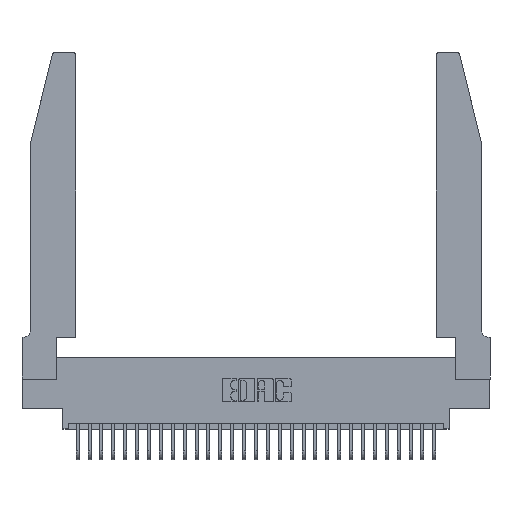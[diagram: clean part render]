
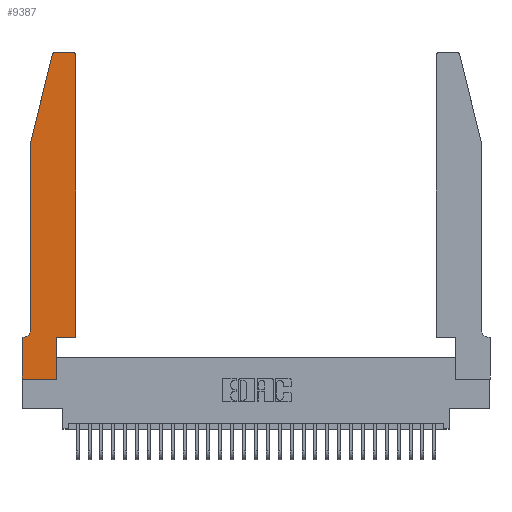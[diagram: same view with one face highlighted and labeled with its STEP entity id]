
A CAD part, top view. The second image highlights one B-rep face of the part: STEP entity #9387.
In plain terms, the highlighted planar face has unit normal (0, 0, 1).
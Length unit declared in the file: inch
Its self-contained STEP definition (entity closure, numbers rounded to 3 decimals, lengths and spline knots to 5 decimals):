
#382 = DIRECTION ( 'NONE',  ( 1., 0., 0. ) ) ;
#825 = CARTESIAN_POINT ( 'NONE',  ( 0.2605, 2.75, 0.37 ) ) ;
#938 = ORIENTED_EDGE ( 'NONE', *, *, #24118, .T. ) ;
#1009 = LINE ( 'NONE', #17457, #20301 ) ;
#1211 = VERTEX_POINT ( 'NONE', #24984 ) ;
#1546 = VERTEX_POINT ( 'NONE', #30286 ) ;
#1888 = ORIENTED_EDGE ( 'NONE', *, *, #3503, .T. ) ;
#2112 = DIRECTION ( 'NONE',  ( 0., 0., -1. ) ) ;
#2207 = CARTESIAN_POINT ( 'NONE',  ( 0.0755, 2., 0.37 ) ) ;
#2732 = VERTEX_POINT ( 'NONE', #14739 ) ;
#3503 = EDGE_CURVE ( 'NONE', #20145, #19215, #1009, .T. ) ;
#3600 = ORIENTED_EDGE ( 'NONE', *, *, #26522, .T. ) ;
#4084 = DIRECTION ( 'NONE',  ( -0.239, -0.971, 0. ) ) ;
#4304 = LINE ( 'NONE', #28898, #10932 ) ;
#5076 = VERTEX_POINT ( 'NONE', #25615 ) ;
#5944 = DIRECTION ( 'NONE',  ( -1., 0., 0. ) ) ;
#6118 = DIRECTION ( 'NONE',  ( 1., 0., 0. ) ) ;
#7181 = ORIENTED_EDGE ( 'NONE', *, *, #22778, .T. ) ;
#7302 = CARTESIAN_POINT ( 'NONE',  ( 0.2865, 0.35, 0.37 ) ) ;
#7409 = LINE ( 'NONE', #26250, #19209 ) ;
#7454 = CARTESIAN_POINT ( 'NONE',  ( 0.284, 2.72, 0.37 ) ) ;
#7634 = EDGE_LOOP ( 'NONE', ( #18173, #3600, #7181, #1888, #30532, #29376, #14653, #9561, #26507, #25388, #938, #20153 ) ) ;
#9213 = AXIS2_PLACEMENT_3D ( 'NONE', #17176, #2112, #19725 ) ;
#9292 = LINE ( 'NONE', #7302, #22596 ) ;
#9387 = ADVANCED_FACE ( 'NONE', ( #9407 ), #18840, .T. ) ;
#9407 = FACE_OUTER_BOUND ( 'NONE', #7634, .T. ) ;
#9561 = ORIENTED_EDGE ( 'NONE', *, *, #23889, .T. ) ;
#9820 = DIRECTION ( 'NONE',  ( 0., 1., 0. ) ) ;
#9963 = DIRECTION ( 'NONE',  ( 1., 0., 0. ) ) ;
#10571 = CARTESIAN_POINT ( 'NONE',  ( 0.25487, 2.72718, 0.37 ) ) ;
#10854 = VERTEX_POINT ( 'NONE', #26149 ) ;
#10932 = VECTOR ( 'NONE', #4084, 39.37008 ) ;
#11085 = EDGE_CURVE ( 'NONE', #19215, #5076, #17549, .T. ) ;
#11135 = EDGE_CURVE ( 'NONE', #1211, #17978, #9292, .T. ) ;
#11339 = DIRECTION ( 'NONE',  ( 1., 0., 0. ) ) ;
#11965 = CIRCLE ( 'NONE', #25156, 0.03 ) ;
#11999 = CARTESIAN_POINT ( 'NONE',  ( 0.4505, 0.35, 0.37 ) ) ;
#12508 = DIRECTION ( 'NONE',  ( 0., -1., 0. ) ) ;
#13237 = VERTEX_POINT ( 'NONE', #10571 ) ;
#13361 = CARTESIAN_POINT ( 'NONE',  ( 0., 0., 0.37 ) ) ;
#14220 = AXIS2_PLACEMENT_3D ( 'NONE', #28624, #26255, #11339 ) ;
#14583 = EDGE_CURVE ( 'NONE', #17978, #18761, #30625, .T. ) ;
#14653 = ORIENTED_EDGE ( 'NONE', *, *, #29157, .T. ) ;
#14739 = CARTESIAN_POINT ( 'NONE',  ( 0., 0.35, 0.37 ) ) ;
#15487 = DIRECTION ( 'NONE',  ( 0., 0., 1. ) ) ;
#16103 = EDGE_CURVE ( 'NONE', #5076, #2732, #20900, .T. ) ;
#17176 = CARTESIAN_POINT ( 'NONE',  ( 0.0055, 0.42, 0.37 ) ) ;
#17457 = CARTESIAN_POINT ( 'NONE',  ( 0.0755, 2., 0.37 ) ) ;
#17549 = CIRCLE ( 'NONE', #9213, 0.07 ) ;
#17978 = VERTEX_POINT ( 'NONE', #18055 ) ;
#18055 = CARTESIAN_POINT ( 'NONE',  ( 0.2865, 0.35, 0.37 ) ) ;
#18173 = ORIENTED_EDGE ( 'NONE', *, *, #18730, .T. ) ;
#18374 = CARTESIAN_POINT ( 'NONE',  ( 0.0755, 0.35, 0.37 ) ) ;
#18466 = VECTOR ( 'NONE', #5944, 39.37008 ) ;
#18730 = EDGE_CURVE ( 'NONE', #1546, #28524, #25031, .T. ) ;
#18761 = VERTEX_POINT ( 'NONE', #30815 ) ;
#18840 = PLANE ( 'NONE',  #14220 ) ;
#19209 = VECTOR ( 'NONE', #28721, 39.37008 ) ;
#19215 = VERTEX_POINT ( 'NONE', #21355 ) ;
#19587 = VECTOR ( 'NONE', #19614, 39.37008 ) ;
#19614 = DIRECTION ( 'NONE',  ( 0., 1., 0. ) ) ;
#19725 = DIRECTION ( 'NONE',  ( -1., 0., 0. ) ) ;
#20145 = VERTEX_POINT ( 'NONE', #2207 ) ;
#20153 = ORIENTED_EDGE ( 'NONE', *, *, #28465, .T. ) ;
#20301 = VECTOR ( 'NONE', #12508, 39.37008 ) ;
#20900 = LINE ( 'NONE', #18374, #26683 ) ;
#21355 = CARTESIAN_POINT ( 'NONE',  ( 0.0755, 0.42, 0.37 ) ) ;
#22040 = CIRCLE ( 'NONE', #28076, 0.03 ) ;
#22596 = VECTOR ( 'NONE', #9820, 39.37008 ) ;
#22778 = EDGE_CURVE ( 'NONE', #13237, #20145, #4304, .T. ) ;
#23889 = EDGE_CURVE ( 'NONE', #32369, #1211, #7409, .T. ) ;
#24095 = VECTOR ( 'NONE', #6118, 39.37008 ) ;
#24118 = EDGE_CURVE ( 'NONE', #18761, #10854, #26881, .T. ) ;
#24911 = DIRECTION ( 'NONE',  ( 0., 0., 1. ) ) ;
#24984 = CARTESIAN_POINT ( 'NONE',  ( 0.2865, 0., 0.37 ) ) ;
#25031 = LINE ( 'NONE', #825, #18466 ) ;
#25156 = AXIS2_PLACEMENT_3D ( 'NONE', #7454, #24911, #9963 ) ;
#25388 = ORIENTED_EDGE ( 'NONE', *, *, #14583, .T. ) ;
#25568 = CARTESIAN_POINT ( 'NONE',  ( 0.284, 2.75, 0.37 ) ) ;
#25615 = CARTESIAN_POINT ( 'NONE',  ( 0.0055, 0.35, 0.37 ) ) ;
#26149 = CARTESIAN_POINT ( 'NONE',  ( 0.4505, 2.72, 0.37 ) ) ;
#26250 = CARTESIAN_POINT ( 'NONE',  ( 0., 0., 0.37 ) ) ;
#26255 = DIRECTION ( 'NONE',  ( 0., 0., 1. ) ) ;
#26507 = ORIENTED_EDGE ( 'NONE', *, *, #11135, .T. ) ;
#26522 = EDGE_CURVE ( 'NONE', #28524, #13237, #11965, .T. ) ;
#26683 = VECTOR ( 'NONE', #28179, 39.37008 ) ;
#26881 = LINE ( 'NONE', #11999, #19587 ) ;
#28076 = AXIS2_PLACEMENT_3D ( 'NONE', #30301, #15487, #382 ) ;
#28179 = DIRECTION ( 'NONE',  ( -1., 0., 0. ) ) ;
#28465 = EDGE_CURVE ( 'NONE', #10854, #1546, #22040, .T. ) ;
#28524 = VERTEX_POINT ( 'NONE', #25568 ) ;
#28624 = CARTESIAN_POINT ( 'NONE',  ( 0., 0.35, 0.37 ) ) ;
#28721 = DIRECTION ( 'NONE',  ( 1., 0., 0. ) ) ;
#28888 = LINE ( 'NONE', #13361, #31207 ) ;
#28898 = CARTESIAN_POINT ( 'NONE',  ( 0.0755, 2., 0.37 ) ) ;
#29157 = EDGE_CURVE ( 'NONE', #2732, #32369, #28888, .T. ) ;
#29376 = ORIENTED_EDGE ( 'NONE', *, *, #16103, .T. ) ;
#30041 = CARTESIAN_POINT ( 'NONE',  ( 0., 0., 0.37 ) ) ;
#30286 = CARTESIAN_POINT ( 'NONE',  ( 0.4205, 2.75, 0.37 ) ) ;
#30301 = CARTESIAN_POINT ( 'NONE',  ( 0.4205, 2.72, 0.37 ) ) ;
#30532 = ORIENTED_EDGE ( 'NONE', *, *, #11085, .T. ) ;
#30625 = LINE ( 'NONE', #30899, #24095 ) ;
#30694 = DIRECTION ( 'NONE',  ( 0., -1., 0. ) ) ;
#30815 = CARTESIAN_POINT ( 'NONE',  ( 0.4505, 0.35, 0.37 ) ) ;
#30899 = CARTESIAN_POINT ( 'NONE',  ( 0.4505, 0.35, 0.37 ) ) ;
#31207 = VECTOR ( 'NONE', #30694, 39.37008 ) ;
#32369 = VERTEX_POINT ( 'NONE', #30041 ) ;
